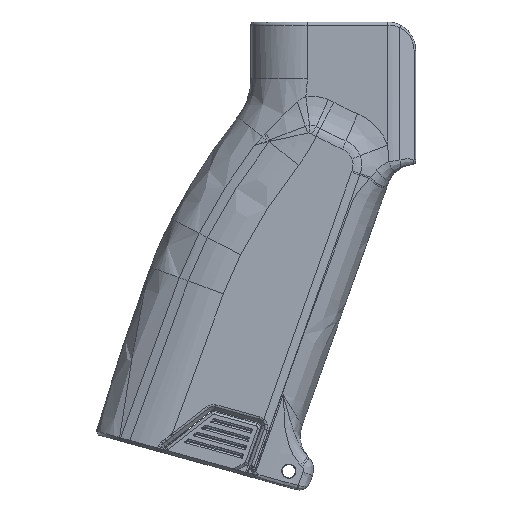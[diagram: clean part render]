
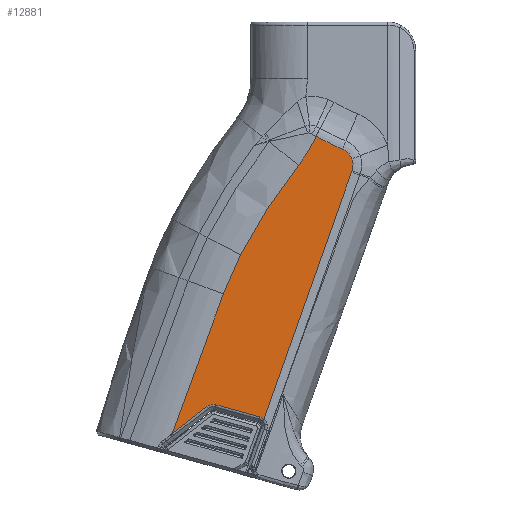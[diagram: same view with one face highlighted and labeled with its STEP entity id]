
A CAD part, left-side view. The second image highlights one B-rep face of the part: STEP entity #12881.
In plain terms, the highlighted planar face has unit normal (-1, 0, 0).
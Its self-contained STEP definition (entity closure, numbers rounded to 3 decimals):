
#923=CIRCLE('',#13678,2.311);
#929=CIRCLE('',#13686,2.311);
#942=CIRCLE('',#13717,3.889);
#943=CIRCLE('',#13718,75.936);
#1482=FACE_OUTER_BOUND('',#2309,.T.);
#2309=EDGE_LOOP('',(#9837,#9838,#9839,#9840,#9841,#9842,#9843,#9844,#9845,
#9846,#9847,#9848,#9849));
#3248=B_SPLINE_CURVE_WITH_KNOTS('',3,(#25704,#25705,#25706,#25707),
 .UNSPECIFIED.,.F.,.F.,(4,4),(-0.031,0.),
 .UNSPECIFIED.);
#3249=B_SPLINE_CURVE_WITH_KNOTS('',3,(#25709,#25710,#25711,#25712),
 .UNSPECIFIED.,.F.,.F.,(4,4),(0.,0.275),.UNSPECIFIED.);
#3250=B_SPLINE_CURVE_WITH_KNOTS('',3,(#25718,#25719,#25720,#25721),
 .UNSPECIFIED.,.F.,.F.,(4,4),(-0.596,0.166),
 .UNSPECIFIED.);
#3251=B_SPLINE_CURVE_WITH_KNOTS('',3,(#25723,#25724,#25725,#25726),
 .UNSPECIFIED.,.F.,.F.,(4,4),(-2.413,0.),.UNSPECIFIED.);
#3252=B_SPLINE_CURVE_WITH_KNOTS('',3,(#25727,#25728,#25729,#25730),
 .UNSPECIFIED.,.F.,.F.,(4,4),(-0.965,0.),.UNSPECIFIED.);
#3556=LINE('',#18418,#4342);
#3743=LINE('',#25304,#4529);
#3745=LINE('',#25316,#4531);
#3758=LINE('',#25595,#4544);
#4342=VECTOR('',#14463,10.);
#4529=VECTOR('',#15132,10.);
#4531=VECTOR('',#15146,10.);
#4544=VECTOR('',#15185,10.);
#5181=VERTEX_POINT('',#18415);
#5182=VERTEX_POINT('',#18417);
#5587=VERTEX_POINT('',#25294);
#5589=VERTEX_POINT('',#25300);
#5591=VERTEX_POINT('',#25306);
#5593=VERTEX_POINT('',#25312);
#5612=VERTEX_POINT('',#25594);
#5625=VERTEX_POINT('',#25703);
#5626=VERTEX_POINT('',#25708);
#5627=VERTEX_POINT('',#25713);
#5628=VERTEX_POINT('',#25715);
#5629=VERTEX_POINT('',#25717);
#5630=VERTEX_POINT('',#25722);
#6412=EDGE_CURVE('',#5181,#5182,#3556,.T.);
#7066=EDGE_CURVE('',#5182,#5587,#923,.T.);
#7071=EDGE_CURVE('',#5587,#5589,#3743,.T.);
#7074=EDGE_CURVE('',#5589,#5591,#929,.T.);
#7077=EDGE_CURVE('',#5591,#5593,#3745,.T.);
#7111=EDGE_CURVE('',#5593,#5612,#3758,.T.);
#7135=EDGE_CURVE('',#5625,#5181,#3248,.T.);
#7136=EDGE_CURVE('',#5626,#5625,#3249,.T.);
#7137=EDGE_CURVE('',#5627,#5626,#942,.T.);
#7138=EDGE_CURVE('',#5628,#5627,#943,.T.);
#7139=EDGE_CURVE('',#5629,#5628,#3250,.T.);
#7140=EDGE_CURVE('',#5630,#5629,#3251,.T.);
#7141=EDGE_CURVE('',#5612,#5630,#3252,.T.);
#9837=ORIENTED_EDGE('',*,*,#7066,.F.);
#9838=ORIENTED_EDGE('',*,*,#6412,.F.);
#9839=ORIENTED_EDGE('',*,*,#7135,.F.);
#9840=ORIENTED_EDGE('',*,*,#7136,.F.);
#9841=ORIENTED_EDGE('',*,*,#7137,.F.);
#9842=ORIENTED_EDGE('',*,*,#7138,.F.);
#9843=ORIENTED_EDGE('',*,*,#7139,.F.);
#9844=ORIENTED_EDGE('',*,*,#7140,.F.);
#9845=ORIENTED_EDGE('',*,*,#7141,.F.);
#9846=ORIENTED_EDGE('',*,*,#7111,.F.);
#9847=ORIENTED_EDGE('',*,*,#7077,.F.);
#9848=ORIENTED_EDGE('',*,*,#7074,.F.);
#9849=ORIENTED_EDGE('',*,*,#7071,.F.);
#12414=PLANE('',#13716);
#12881=ADVANCED_FACE('',(#1482),#12414,.T.);
#13678=AXIS2_PLACEMENT_3D('',#25295,#15121,#15122);
#13686=AXIS2_PLACEMENT_3D('',#25310,#15139,#15140);
#13716=AXIS2_PLACEMENT_3D('',#25702,#15224,#15225);
#13717=AXIS2_PLACEMENT_3D('',#25714,#15226,#15227);
#13718=AXIS2_PLACEMENT_3D('',#25716,#15228,#15229);
#14463=DIRECTION('',(0.,0.335,-0.942));
#15121=DIRECTION('center_axis',(-1.,0.,0.));
#15122=DIRECTION('ref_axis',(0.,-0.499,0.867));
#15132=DIRECTION('',(0.,0.964,0.266));
#15139=DIRECTION('center_axis',(-1.,0.,0.));
#15140=DIRECTION('ref_axis',(0.,0.194,0.981));
#15146=DIRECTION('',(0.,0.79,-0.613));
#15185=DIRECTION('',(0.,-0.344,0.939));
#15224=DIRECTION('center_axis',(-1.,0.,0.));
#15225=DIRECTION('ref_axis',(0.,-1.,0.));
#15226=DIRECTION('center_axis',(1.,0.,0.));
#15227=DIRECTION('ref_axis',(0.,-0.72,0.694));
#15228=DIRECTION('center_axis',(-1.,0.,0.));
#15229=DIRECTION('ref_axis',(0.,0.433,-0.901));
#18415=CARTESIAN_POINT('',(-13.29,-139.811,-43.074));
#18417=CARTESIAN_POINT('',(-13.29,-119.985,-98.836));
#18418=CARTESIAN_POINT('',(-13.29,-123.761,-88.216));
#25294=CARTESIAN_POINT('',(-13.29,-119.086,-98.354));
#25295=CARTESIAN_POINT('Origin',(-13.29,-118.471,-100.581));
#25300=CARTESIAN_POINT('',(-13.29,-109.196,-95.624));
#25304=CARTESIAN_POINT('',(-13.29,-111.571,-96.279));
#25306=CARTESIAN_POINT('',(-13.29,-107.164,-96.026));
#25310=CARTESIAN_POINT('Origin',(-13.29,-108.581,-97.851));
#25312=CARTESIAN_POINT('',(-13.29,-99.336,-102.103));
#25316=CARTESIAN_POINT('',(-13.29,-126.252,-81.205));
#25594=CARTESIAN_POINT('',(-13.29,-110.892,-70.588));
#25595=CARTESIAN_POINT('',(-13.29,-110.892,-70.588));
#25702=CARTESIAN_POINT('Origin',(-13.29,-121.21,-61.501));
#25703=CARTESIAN_POINT('',(-13.29,-139.915,-42.781));
#25704=CARTESIAN_POINT('Ctrl Pts',(-13.29,-139.915,
-42.781));
#25705=CARTESIAN_POINT('Ctrl Pts',(-13.29,-139.88,
-42.879));
#25706=CARTESIAN_POINT('Ctrl Pts',(-13.29,-139.845,
-42.977));
#25707=CARTESIAN_POINT('Ctrl Pts',(-13.29,-139.811,
-43.074));
#25708=CARTESIAN_POINT('',(-13.29,-139.883,-40.083));
#25709=CARTESIAN_POINT('Ctrl Pts',(-13.29,-139.883,-40.083));
#25710=CARTESIAN_POINT('Ctrl Pts',(-13.29,-140.212,
-40.94));
#25711=CARTESIAN_POINT('Ctrl Pts',(-13.29,-140.222,
-41.916));
#25712=CARTESIAN_POINT('Ctrl Pts',(-13.29,-139.915,
-42.781));
#25713=CARTESIAN_POINT('',(-13.29,-137.78,-37.898));
#25714=CARTESIAN_POINT('Origin',(-13.29,-136.252,-41.474));
#25715=CARTESIAN_POINT('',(-13.29,-131.81,-35.034));
#25716=CARTESIAN_POINT('Origin',(-13.29,-167.611,31.933));
#25717=CARTESIAN_POINT('',(-13.29,-127.852,-41.526));
#25718=CARTESIAN_POINT('Ctrl Pts',(-13.29,-127.852,
-41.526));
#25719=CARTESIAN_POINT('Ctrl Pts',(-13.29,-129.427,-39.533));
#25720=CARTESIAN_POINT('Ctrl Pts',(-13.29,-130.759,
-37.348));
#25721=CARTESIAN_POINT('Ctrl Pts',(-13.29,-131.81,
-35.034));
#25722=CARTESIAN_POINT('',(-13.29,-114.781,-61.762));
#25723=CARTESIAN_POINT('Ctrl Pts',(-13.29,-114.781,
-61.762));
#25724=CARTESIAN_POINT('Ctrl Pts',(-13.29,-118.484,
-54.623));
#25725=CARTESIAN_POINT('Ctrl Pts',(-13.29,-122.867,
-47.837));
#25726=CARTESIAN_POINT('Ctrl Pts',(-13.29,-127.852,
-41.526));
#25727=CARTESIAN_POINT('Ctrl Pts',(-13.29,-110.892,
-70.588));
#25728=CARTESIAN_POINT('Ctrl Pts',(-13.29,-111.999,
-67.568));
#25729=CARTESIAN_POINT('Ctrl Pts',(-13.29,-113.299,
-64.618));
#25730=CARTESIAN_POINT('Ctrl Pts',(-13.29,-114.781,
-61.762));
